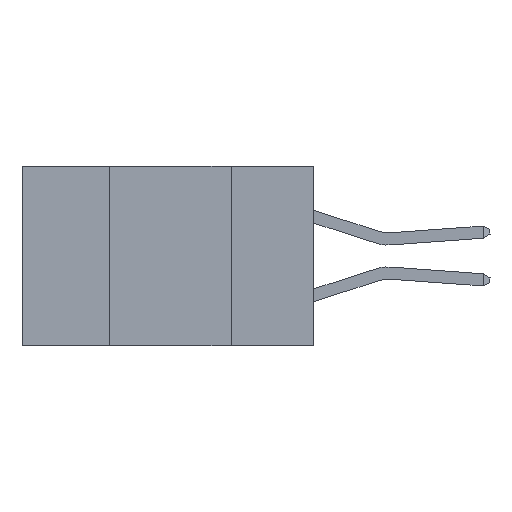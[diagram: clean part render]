
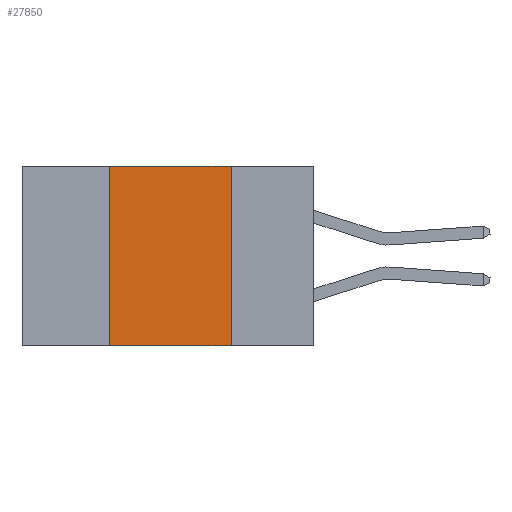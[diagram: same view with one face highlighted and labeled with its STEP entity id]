
A CAD part, left-side view. The second image highlights one B-rep face of the part: STEP entity #27850.
In plain terms, the highlighted planar face has unit normal (-1, 0, 0).
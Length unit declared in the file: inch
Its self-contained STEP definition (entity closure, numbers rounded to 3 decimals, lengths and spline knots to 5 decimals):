
#223 = VERTEX_POINT ( 'NONE', #16533 ) ;
#607 = CARTESIAN_POINT ( 'NONE',  ( 0., 0.6, -0.37 ) ) ;
#971 = EDGE_CURVE ( 'NONE', #31683, #32284, #31629, .T. ) ;
#4623 = EDGE_CURVE ( 'NONE', #223, #32284, #8049, .T. ) ;
#5457 = CARTESIAN_POINT ( 'NONE',  ( 0., 0.17, -0.37 ) ) ;
#6144 = DIRECTION ( 'NONE',  ( 0., -1., 0. ) ) ;
#8049 = LINE ( 'NONE', #607, #12907 ) ;
#12645 = VECTOR ( 'NONE', #19121, 39.37008 ) ;
#12907 = VECTOR ( 'NONE', #6144, 39.37008 ) ;
#13017 = ORIENTED_EDGE ( 'NONE', *, *, #971, .F. ) ;
#13259 = LINE ( 'NONE', #29182, #25973 ) ;
#13288 = CARTESIAN_POINT ( 'NONE',  ( 0., 0.42, 0. ) ) ;
#14111 = EDGE_CURVE ( 'NONE', #32034, #31683, #27596, .T. ) ;
#14175 = DIRECTION ( 'NONE',  ( 0., 0., -1. ) ) ;
#16533 = CARTESIAN_POINT ( 'NONE',  ( 0., 0.42, -0.37 ) ) ;
#16787 = VECTOR ( 'NONE', #14175, 39.37008 ) ;
#19121 = DIRECTION ( 'NONE',  ( 0., -1., 0. ) ) ;
#20404 = FACE_OUTER_BOUND ( 'NONE', #34490, .T. ) ;
#22234 = PLANE ( 'NONE',  #23977 ) ;
#22344 = DIRECTION ( 'NONE',  ( 0., 0., -1. ) ) ;
#23159 = EDGE_CURVE ( 'NONE', #223, #32034, #13259, .T. ) ;
#23219 = ORIENTED_EDGE ( 'NONE', *, *, #4623, .T. ) ;
#23977 = AXIS2_PLACEMENT_3D ( 'NONE', #32951, #27613, #22344 ) ;
#24382 = CARTESIAN_POINT ( 'NONE',  ( 0., 0.17, 0. ) ) ;
#24482 = ORIENTED_EDGE ( 'NONE', *, *, #14111, .F. ) ;
#25973 = VECTOR ( 'NONE', #31959, 39.37008 ) ;
#27330 = CARTESIAN_POINT ( 'NONE',  ( 0., 0.6, 0. ) ) ;
#27596 = LINE ( 'NONE', #27330, #12645 ) ;
#27613 = DIRECTION ( 'NONE',  ( 1., 0., 0. ) ) ;
#27850 = ADVANCED_FACE ( 'NONE', ( #20404 ), #22234, .F. ) ;
#29182 = CARTESIAN_POINT ( 'NONE',  ( 0., 0.42, 0. ) ) ;
#30912 = CARTESIAN_POINT ( 'NONE',  ( 0., 0.17, 0. ) ) ;
#31629 = LINE ( 'NONE', #30912, #16787 ) ;
#31683 = VERTEX_POINT ( 'NONE', #24382 ) ;
#31959 = DIRECTION ( 'NONE',  ( 0., 0., 1. ) ) ;
#32034 = VERTEX_POINT ( 'NONE', #13288 ) ;
#32284 = VERTEX_POINT ( 'NONE', #5457 ) ;
#32951 = CARTESIAN_POINT ( 'NONE',  ( 0., 0.6, 0. ) ) ;
#34490 = EDGE_LOOP ( 'NONE', ( #13017, #24482, #35187, #23219 ) ) ;
#35187 = ORIENTED_EDGE ( 'NONE', *, *, #23159, .F. ) ;
